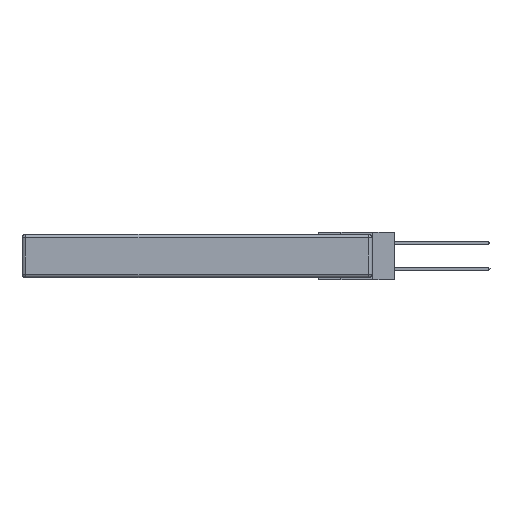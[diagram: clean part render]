
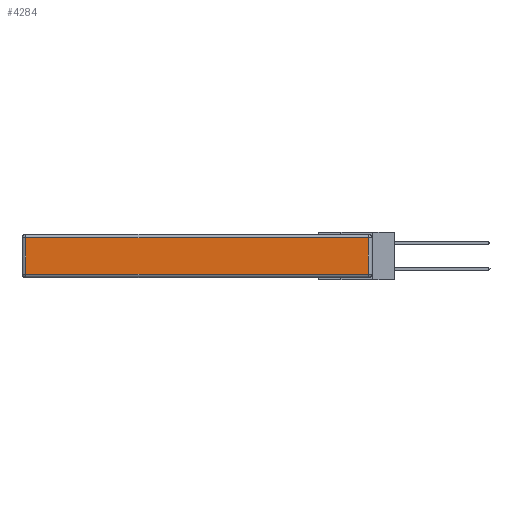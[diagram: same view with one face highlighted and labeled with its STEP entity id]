
A CAD part, left-side view. The second image highlights one B-rep face of the part: STEP entity #4284.
In plain terms, the highlighted planar face has unit normal (-1, 0, 0).
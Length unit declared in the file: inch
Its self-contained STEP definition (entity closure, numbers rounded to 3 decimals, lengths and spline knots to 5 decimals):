
#1456 = CARTESIAN_POINT ( 'NONE',  ( 0., 0.03, -0.03 ) ) ;
#1699 = CARTESIAN_POINT ( 'NONE',  ( 0., 0.03, -0.313 ) ) ;
#1746 = DIRECTION ( 'NONE',  ( -1., 0., 0. ) ) ;
#2105 = DIRECTION ( 'NONE',  ( 0., 1., 0. ) ) ;
#3326 = LINE ( 'NONE', #29810, #14296 ) ;
#4073 = EDGE_CURVE ( 'NONE', #17782, #24462, #15318, .T. ) ;
#4284 = ADVANCED_FACE ( 'NONE', ( #22554 ), #29342, .T. ) ;
#4340 = CARTESIAN_POINT ( 'NONE',  ( 0., 2.75, -0.03 ) ) ;
#4381 = DIRECTION ( 'NONE',  ( 0., 0., 1. ) ) ;
#4799 = ORIENTED_EDGE ( 'NONE', *, *, #26590, .T. ) ;
#8382 = DIRECTION ( 'NONE',  ( 0., -1., 0. ) ) ;
#9420 = EDGE_CURVE ( 'NONE', #23729, #17782, #28516, .T. ) ;
#9434 = LINE ( 'NONE', #15727, #17476 ) ;
#11944 = CARTESIAN_POINT ( 'NONE',  ( 0., 0.03, -0.343 ) ) ;
#14296 = VECTOR ( 'NONE', #16218, 39.37008 ) ;
#15038 = EDGE_CURVE ( 'NONE', #28124, #23729, #9434, .T. ) ;
#15318 = LINE ( 'NONE', #4340, #15639 ) ;
#15639 = VECTOR ( 'NONE', #2105, 39.37008 ) ;
#15727 = CARTESIAN_POINT ( 'NONE',  ( 0., 0., -0.313 ) ) ;
#16127 = ORIENTED_EDGE ( 'NONE', *, *, #4073, .T. ) ;
#16218 = DIRECTION ( 'NONE',  ( 0., 0., -1. ) ) ;
#16235 = ORIENTED_EDGE ( 'NONE', *, *, #15038, .T. ) ;
#17476 = VECTOR ( 'NONE', #8382, 39.37008 ) ;
#17782 = VERTEX_POINT ( 'NONE', #1456 ) ;
#21888 = AXIS2_PLACEMENT_3D ( 'NONE', #24855, #1746, #4381 ) ;
#22259 = EDGE_LOOP ( 'NONE', ( #16235, #22367, #16127, #4799 ) ) ;
#22367 = ORIENTED_EDGE ( 'NONE', *, *, #9420, .T. ) ;
#22554 = FACE_OUTER_BOUND ( 'NONE', #22259, .T. ) ;
#23729 = VERTEX_POINT ( 'NONE', #1699 ) ;
#24462 = VERTEX_POINT ( 'NONE', #27758 ) ;
#24829 = VECTOR ( 'NONE', #27968, 39.37008 ) ;
#24855 = CARTESIAN_POINT ( 'NONE',  ( 0., 0., -0.343 ) ) ;
#26590 = EDGE_CURVE ( 'NONE', #24462, #28124, #3326, .T. ) ;
#27758 = CARTESIAN_POINT ( 'NONE',  ( 0., 2.72, -0.03 ) ) ;
#27968 = DIRECTION ( 'NONE',  ( 0., 0., 1. ) ) ;
#28124 = VERTEX_POINT ( 'NONE', #30023 ) ;
#28516 = LINE ( 'NONE', #11944, #24829 ) ;
#29342 = PLANE ( 'NONE',  #21888 ) ;
#29810 = CARTESIAN_POINT ( 'NONE',  ( 0., 2.72, -0.343 ) ) ;
#30023 = CARTESIAN_POINT ( 'NONE',  ( 0., 2.72, -0.313 ) ) ;
